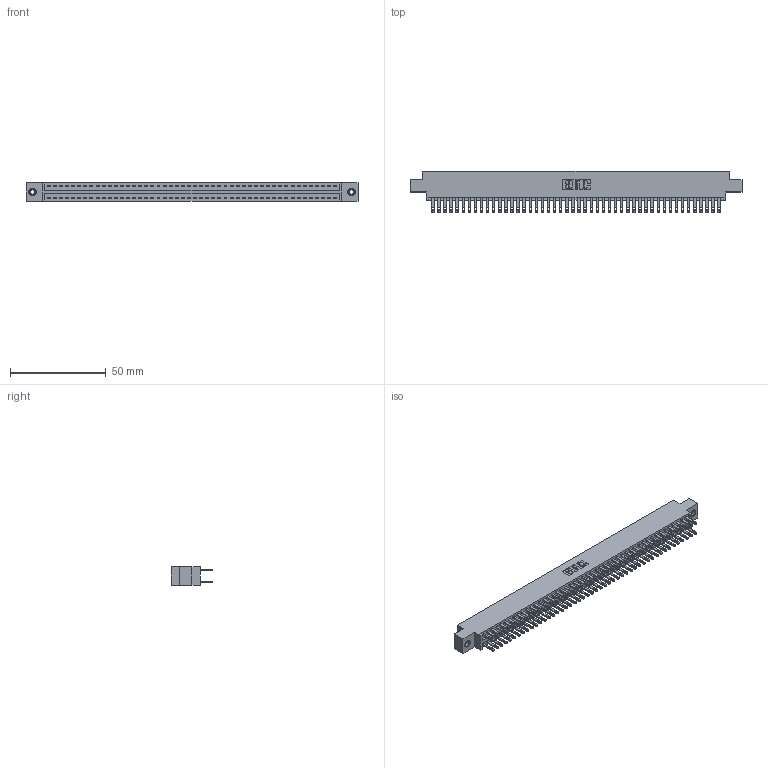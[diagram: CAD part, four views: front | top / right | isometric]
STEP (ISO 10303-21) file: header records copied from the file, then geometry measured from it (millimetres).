
FILE_DESCRIPTION (( 'STEP AP203' ), '1' );
FILE_NAME ('346-096-500-808.STEP', '2018-08-30T06:21:32', ( '' ), ( '' ), 'SwSTEP 2.0', 'SolidWorks 2016', '' );
FILE_SCHEMA (( 'CONFIG_CONTROL_DESIGN' ));
Length unit declared in the file: inch
Products named in the file (4): 346 Part_0.170 Offset - 0.156 Dia-TI; 345-292-001_345-293-100; 345-250-001_345-250-003-102; 346-096-500-808
Assembly tree (99 placements, depth 2):
  346-096-500-808
    346 Part_0.170 Offset - 0.156 Dia-TI
    345-292-001_345-293-100  x96
    345-250-001_345-250-003-102  x2
Bounding box: 172.97 x 21.84 x 9.4 mm (x, y, z)
Volume: 17045.9 mm3; surface area: 24729.5 mm2
Topology: 99 solids, 99 shells, 4794 faces, 14589 edges, 9718 vertices
Faces by surface type: plane 2896, cylinder 1882, cone 12, torus 4
Entity records: 31766 total; most frequent: CARTESIAN_POINT 5211, ORIENTED_EDGE 5138, DIRECTION 4671, EDGE_CURVE 2569, LINE 2221, VECTOR 2221, VERTEX_POINT 1708, AXIS2_PLACEMENT_3D 1225
